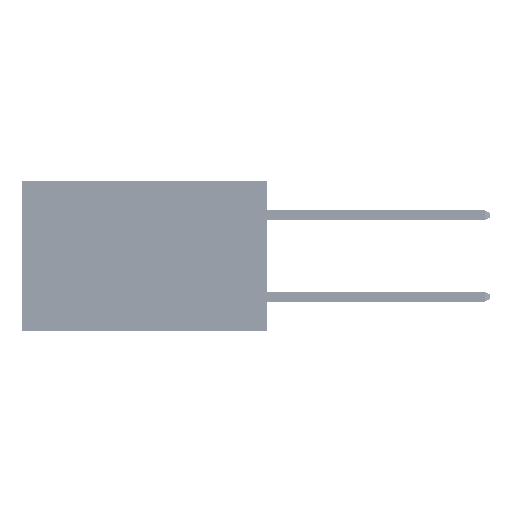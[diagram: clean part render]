
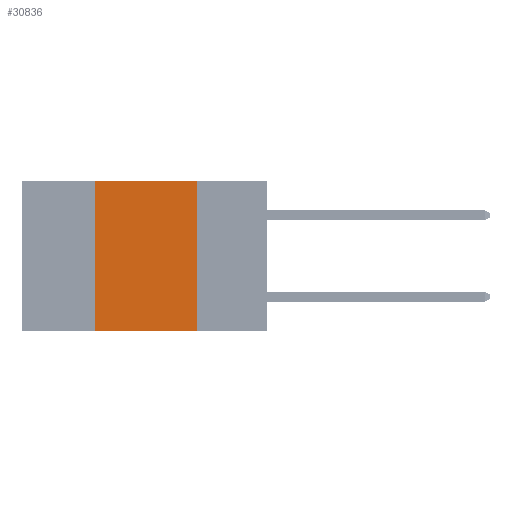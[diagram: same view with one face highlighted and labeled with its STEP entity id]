
A CAD part, left-side view. The second image highlights one B-rep face of the part: STEP entity #30836.
In plain terms, the highlighted planar face has unit normal (-1, 0, 0).
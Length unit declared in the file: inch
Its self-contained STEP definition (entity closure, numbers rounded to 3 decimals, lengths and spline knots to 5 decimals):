
#1792 = CARTESIAN_POINT ( 'NONE',  ( 0., 0.42, -0.37 ) ) ;
#8162 = EDGE_CURVE ( 'NONE', #44782, #26364, #20575, .T. ) ;
#9748 = CARTESIAN_POINT ( 'NONE',  ( 0., 0.42, 0. ) ) ;
#10202 = CARTESIAN_POINT ( 'NONE',  ( 0., 0.42, 0. ) ) ;
#12046 = EDGE_CURVE ( 'NONE', #44782, #24962, #28280, .T. ) ;
#16380 = AXIS2_PLACEMENT_3D ( 'NONE', #43745, #35759, #32060 ) ;
#19983 = EDGE_CURVE ( 'NONE', #24962, #23456, #44943, .T. ) ;
#20259 = FACE_OUTER_BOUND ( 'NONE', #22938, .T. ) ;
#20575 = LINE ( 'NONE', #45136, #40260 ) ;
#22326 = DIRECTION ( 'NONE',  ( 0., -1., 0. ) ) ;
#22938 = EDGE_LOOP ( 'NONE', ( #47244, #24808, #26791, #36912 ) ) ;
#23456 = VERTEX_POINT ( 'NONE', #38502 ) ;
#24808 = ORIENTED_EDGE ( 'NONE', *, *, #19983, .F. ) ;
#24962 = VERTEX_POINT ( 'NONE', #9748 ) ;
#26364 = VERTEX_POINT ( 'NONE', #33189 ) ;
#26791 = ORIENTED_EDGE ( 'NONE', *, *, #12046, .F. ) ;
#27690 = VECTOR ( 'NONE', #42543, 39.37008 ) ;
#28280 = LINE ( 'NONE', #10202, #41367 ) ;
#30836 = ADVANCED_FACE ( 'NONE', ( #20259 ), #31891, .F. ) ;
#31891 = PLANE ( 'NONE',  #16380 ) ;
#32060 = DIRECTION ( 'NONE',  ( 0., 0., -1. ) ) ;
#33189 = CARTESIAN_POINT ( 'NONE',  ( 0., 0.17, -0.37 ) ) ;
#34726 = CARTESIAN_POINT ( 'NONE',  ( 0., 0.17, 0. ) ) ;
#35759 = DIRECTION ( 'NONE',  ( 1., 0., 0. ) ) ;
#36010 = VECTOR ( 'NONE', #36139, 39.37008 ) ;
#36139 = DIRECTION ( 'NONE',  ( 0., -1., 0. ) ) ;
#36912 = ORIENTED_EDGE ( 'NONE', *, *, #8162, .T. ) ;
#38502 = CARTESIAN_POINT ( 'NONE',  ( 0., 0.17, 0. ) ) ;
#40260 = VECTOR ( 'NONE', #22326, 39.37008 ) ;
#40690 = DIRECTION ( 'NONE',  ( 0., 0., 1. ) ) ;
#40831 = EDGE_CURVE ( 'NONE', #23456, #26364, #48559, .T. ) ;
#41367 = VECTOR ( 'NONE', #40690, 39.37008 ) ;
#42543 = DIRECTION ( 'NONE',  ( 0., 0., -1. ) ) ;
#43745 = CARTESIAN_POINT ( 'NONE',  ( 0., 0.6, 0. ) ) ;
#44119 = CARTESIAN_POINT ( 'NONE',  ( 0., 0.6, 0. ) ) ;
#44782 = VERTEX_POINT ( 'NONE', #1792 ) ;
#44943 = LINE ( 'NONE', #44119, #36010 ) ;
#45136 = CARTESIAN_POINT ( 'NONE',  ( 0., 0.6, -0.37 ) ) ;
#47244 = ORIENTED_EDGE ( 'NONE', *, *, #40831, .F. ) ;
#48559 = LINE ( 'NONE', #34726, #27690 ) ;
